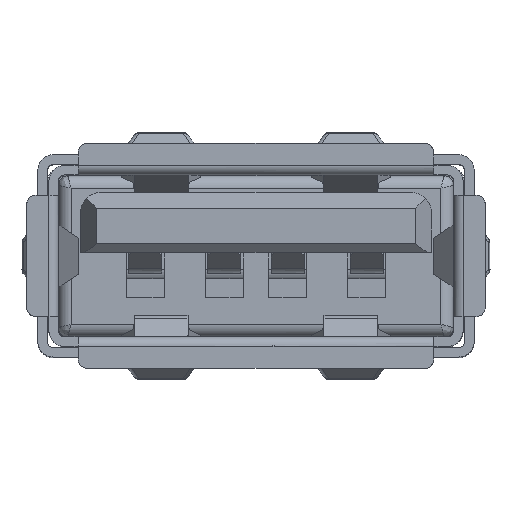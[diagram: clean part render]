
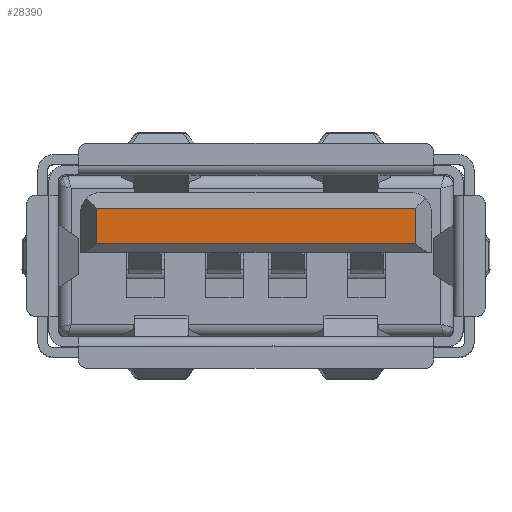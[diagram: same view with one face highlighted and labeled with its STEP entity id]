
A CAD part, top view. The second image highlights one B-rep face of the part: STEP entity #28390.
In plain terms, the highlighted face is planar.
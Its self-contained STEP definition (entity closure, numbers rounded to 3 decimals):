
#1021 = PLANE ( 'NONE',  #23975 ) ;
#3954 = LINE ( 'NONE', #20464, #11225 ) ;
#5802 = CARTESIAN_POINT ( 'NONE',  ( 861.205, 607.953, -4.36 ) ) ;
#7787 = ORIENTED_EDGE ( 'NONE', *, *, #18873, .T. ) ;
#8642 = DIRECTION ( 'NONE',  ( 1., 0., 0. ) ) ;
#9101 = LINE ( 'NONE', #22706, #20658 ) ;
#9255 = EDGE_LOOP ( 'NONE', ( #16498, #13807, #7787, #29392 ) ) ;
#9420 = VERTEX_POINT ( 'NONE', #25560 ) ;
#9594 = LINE ( 'NONE', #30294, #26391 ) ;
#9987 = CARTESIAN_POINT ( 'NONE',  ( 860.705, 607.953, -3.23 ) ) ;
#10353 = CARTESIAN_POINT ( 'NONE',  ( 860.705, 607.953, -3.795 ) ) ;
#10934 = EDGE_CURVE ( 'NONE', #12334, #27043, #20069, .T. ) ;
#11042 = VERTEX_POINT ( 'NONE', #27742 ) ;
#11225 = VECTOR ( 'NONE', #25714, 1000. ) ;
#11933 = VECTOR ( 'NONE', #12971, 1000. ) ;
#12334 = VERTEX_POINT ( 'NONE', #27002 ) ;
#12971 = DIRECTION ( 'NONE',  ( 0., 0., 1. ) ) ;
#13807 = ORIENTED_EDGE ( 'NONE', *, *, #25113, .T. ) ;
#16238 = DIRECTION ( 'NONE',  ( 0., 0., 1. ) ) ;
#16498 = ORIENTED_EDGE ( 'NONE', *, *, #29406, .F. ) ;
#18873 = EDGE_CURVE ( 'NONE', #9420, #27043, #9101, .T. ) ;
#20069 = LINE ( 'NONE', #10353, #11933 ) ;
#20464 = CARTESIAN_POINT ( 'NONE',  ( 861.205, 607.953, -4.36 ) ) ;
#20658 = VECTOR ( 'NONE', #8642, 1000. ) ;
#22195 = FACE_OUTER_BOUND ( 'NONE', #9255, .T. ) ;
#22706 = CARTESIAN_POINT ( 'NONE',  ( 861.205, 607.953, -3.23 ) ) ;
#23102 = DIRECTION ( 'NONE',  ( 0., 0., 1. ) ) ;
#23975 = AXIS2_PLACEMENT_3D ( 'NONE', #5802, #29898, #23102 ) ;
#25113 = EDGE_CURVE ( 'NONE', #11042, #9420, #9594, .T. ) ;
#25560 = CARTESIAN_POINT ( 'NONE',  ( 850.605, 607.953, -3.23 ) ) ;
#25714 = DIRECTION ( 'NONE',  ( 1., 0., 0. ) ) ;
#26391 = VECTOR ( 'NONE', #16238, 1000. ) ;
#27002 = CARTESIAN_POINT ( 'NONE',  ( 860.705, 607.953, -4.36 ) ) ;
#27043 = VERTEX_POINT ( 'NONE', #9987 ) ;
#27742 = CARTESIAN_POINT ( 'NONE',  ( 850.605, 607.953, -4.36 ) ) ;
#28390 = ADVANCED_FACE ( 'NONE', ( #22195 ), #1021, .T. ) ;
#29392 = ORIENTED_EDGE ( 'NONE', *, *, #10934, .F. ) ;
#29406 = EDGE_CURVE ( 'NONE', #11042, #12334, #3954, .T. ) ;
#29898 = DIRECTION ( 'NONE',  ( 0., 1., 0. ) ) ;
#30294 = CARTESIAN_POINT ( 'NONE',  ( 850.605, 607.953, -4.36 ) ) ;
